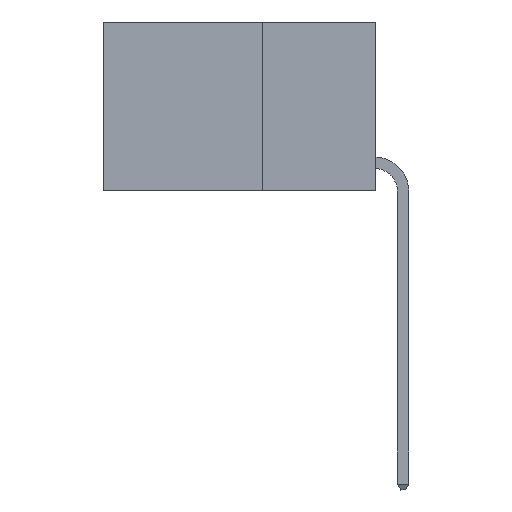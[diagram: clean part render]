
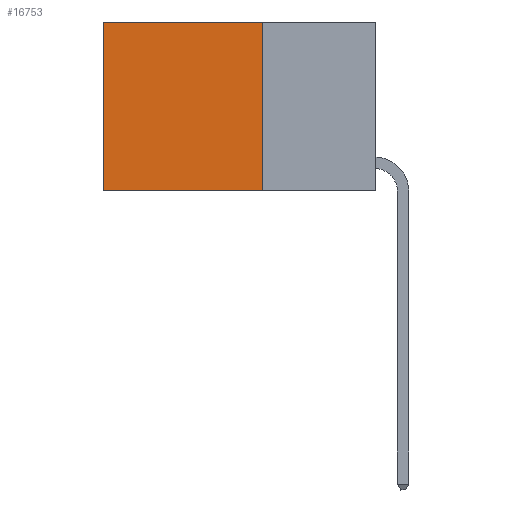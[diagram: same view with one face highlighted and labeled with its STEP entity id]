
A CAD part, left-side view. The second image highlights one B-rep face of the part: STEP entity #16753.
In plain terms, the highlighted planar face has unit normal (-1, 0, 0).
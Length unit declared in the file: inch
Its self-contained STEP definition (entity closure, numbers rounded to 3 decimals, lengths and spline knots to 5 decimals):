
#13 = PLANE ( 'NONE',  #6334 ) ;
#762 = CARTESIAN_POINT ( 'NONE',  ( 0.2625, 0.25, 0. ) ) ;
#1679 = DIRECTION ( 'NONE',  ( 0., 0., -1. ) ) ;
#1963 = CARTESIAN_POINT ( 'NONE',  ( 0.2625, 0.6, 0. ) ) ;
#2342 = VECTOR ( 'NONE', #10937, 39.37008 ) ;
#2740 = LINE ( 'NONE', #15368, #5236 ) ;
#3001 = EDGE_CURVE ( 'NONE', #16644, #5657, #14665, .T. ) ;
#4114 = VECTOR ( 'NONE', #17162, 39.37008 ) ;
#4290 = ORIENTED_EDGE ( 'NONE', *, *, #3001, .T. ) ;
#5133 = EDGE_LOOP ( 'NONE', ( #4290, #17075, #14237, #12032 ) ) ;
#5236 = VECTOR ( 'NONE', #16768, 39.37008 ) ;
#5657 = VERTEX_POINT ( 'NONE', #15031 ) ;
#6085 = CARTESIAN_POINT ( 'NONE',  ( 0.2625, 0.25, -0.37 ) ) ;
#6334 = AXIS2_PLACEMENT_3D ( 'NONE', #8743, #7158, #1679 ) ;
#6643 = EDGE_CURVE ( 'NONE', #8245, #10236, #2740, .T. ) ;
#7158 = DIRECTION ( 'NONE',  ( 1., 0., 0. ) ) ;
#7249 = FACE_OUTER_BOUND ( 'NONE', #5133, .T. ) ;
#8170 = CARTESIAN_POINT ( 'NONE',  ( 0.2625, 0.6, 0. ) ) ;
#8245 = VERTEX_POINT ( 'NONE', #9105 ) ;
#8743 = CARTESIAN_POINT ( 'NONE',  ( 0.2625, 0.25, 0. ) ) ;
#9105 = CARTESIAN_POINT ( 'NONE',  ( 0.2625, 0.25, 0. ) ) ;
#9149 = LINE ( 'NONE', #762, #10275 ) ;
#9777 = EDGE_CURVE ( 'NONE', #10236, #5657, #14548, .T. ) ;
#10236 = VERTEX_POINT ( 'NONE', #13051 ) ;
#10275 = VECTOR ( 'NONE', #13762, 39.37008 ) ;
#10937 = DIRECTION ( 'NONE',  ( 0., 0., -1. ) ) ;
#12032 = ORIENTED_EDGE ( 'NONE', *, *, #17791, .T. ) ;
#13051 = CARTESIAN_POINT ( 'NONE',  ( 0.2625, 0.25, -0.37 ) ) ;
#13762 = DIRECTION ( 'NONE',  ( 0., 1., 0. ) ) ;
#14237 = ORIENTED_EDGE ( 'NONE', *, *, #6643, .F. ) ;
#14548 = LINE ( 'NONE', #6085, #4114 ) ;
#14665 = LINE ( 'NONE', #1963, #2342 ) ;
#15031 = CARTESIAN_POINT ( 'NONE',  ( 0.2625, 0.6, -0.37 ) ) ;
#15368 = CARTESIAN_POINT ( 'NONE',  ( 0.2625, 0.25, 0. ) ) ;
#16644 = VERTEX_POINT ( 'NONE', #8170 ) ;
#16753 = ADVANCED_FACE ( 'NONE', ( #7249 ), #13, .F. ) ;
#16768 = DIRECTION ( 'NONE',  ( 0., 0., -1. ) ) ;
#17075 = ORIENTED_EDGE ( 'NONE', *, *, #9777, .F. ) ;
#17162 = DIRECTION ( 'NONE',  ( 0., 1., 0. ) ) ;
#17791 = EDGE_CURVE ( 'NONE', #8245, #16644, #9149, .T. ) ;
